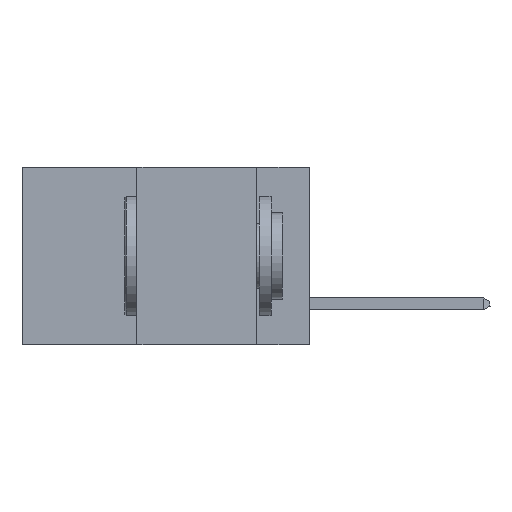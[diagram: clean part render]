
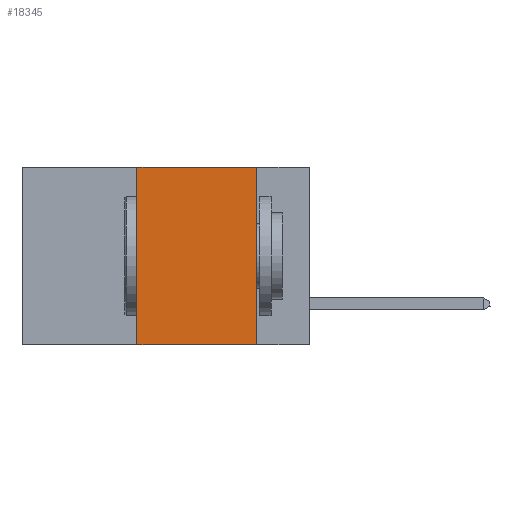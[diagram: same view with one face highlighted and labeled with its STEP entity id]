
A CAD part, left-side view. The second image highlights one B-rep face of the part: STEP entity #18345.
In plain terms, the highlighted planar face has unit normal (-1, 0, 0).
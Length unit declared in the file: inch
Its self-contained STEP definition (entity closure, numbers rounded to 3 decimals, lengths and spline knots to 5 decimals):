
#171 = VERTEX_POINT ( 'NONE', #15645 ) ;
#567 = CARTESIAN_POINT ( 'NONE',  ( 0., 0.36, 0. ) ) ;
#856 = CARTESIAN_POINT ( 'NONE',  ( 0., 0.6, 0. ) ) ;
#2306 = ORIENTED_EDGE ( 'NONE', *, *, #4148, .F. ) ;
#2376 = EDGE_LOOP ( 'NONE', ( #21648, #2306, #12618, #24026 ) ) ;
#2383 = LINE ( 'NONE', #19832, #6297 ) ;
#2520 = DIRECTION ( 'NONE',  ( 0., 0., 1. ) ) ;
#2818 = DIRECTION ( 'NONE',  ( 0., 0., -1. ) ) ;
#4148 = EDGE_CURVE ( 'NONE', #15602, #171, #2383, .T. ) ;
#4339 = CARTESIAN_POINT ( 'NONE',  ( 0., 0.11, 0. ) ) ;
#4384 = VERTEX_POINT ( 'NONE', #9303 ) ;
#5113 = CARTESIAN_POINT ( 'NONE',  ( 0., 0.6, -0.37 ) ) ;
#6297 = VECTOR ( 'NONE', #19319, 39.37008 ) ;
#7055 = DIRECTION ( 'NONE',  ( 0., -1., 0. ) ) ;
#9303 = CARTESIAN_POINT ( 'NONE',  ( 0., 0.11, -0.37 ) ) ;
#9849 = EDGE_CURVE ( 'NONE', #18872, #4384, #13884, .T. ) ;
#10145 = AXIS2_PLACEMENT_3D ( 'NONE', #856, #14444, #2818 ) ;
#11339 = EDGE_CURVE ( 'NONE', #18872, #15602, #24880, .T. ) ;
#12463 = CARTESIAN_POINT ( 'NONE',  ( 0., 0.36, -0.37 ) ) ;
#12618 = ORIENTED_EDGE ( 'NONE', *, *, #11339, .F. ) ;
#13273 = VECTOR ( 'NONE', #7055, 39.37008 ) ;
#13844 = VECTOR ( 'NONE', #2520, 39.37008 ) ;
#13884 = LINE ( 'NONE', #5113, #13273 ) ;
#14359 = FACE_OUTER_BOUND ( 'NONE', #2376, .T. ) ;
#14444 = DIRECTION ( 'NONE',  ( 1., 0., 0. ) ) ;
#15079 = EDGE_CURVE ( 'NONE', #171, #4384, #20224, .T. ) ;
#15127 = VECTOR ( 'NONE', #21736, 39.37008 ) ;
#15602 = VERTEX_POINT ( 'NONE', #24952 ) ;
#15645 = CARTESIAN_POINT ( 'NONE',  ( 0., 0.11, 0. ) ) ;
#18345 = ADVANCED_FACE ( 'NONE', ( #14359 ), #22078, .F. ) ;
#18872 = VERTEX_POINT ( 'NONE', #12463 ) ;
#19319 = DIRECTION ( 'NONE',  ( 0., -1., 0. ) ) ;
#19832 = CARTESIAN_POINT ( 'NONE',  ( 0., 0.6, 0. ) ) ;
#20224 = LINE ( 'NONE', #4339, #15127 ) ;
#21648 = ORIENTED_EDGE ( 'NONE', *, *, #15079, .F. ) ;
#21736 = DIRECTION ( 'NONE',  ( 0., 0., -1. ) ) ;
#22078 = PLANE ( 'NONE',  #10145 ) ;
#24026 = ORIENTED_EDGE ( 'NONE', *, *, #9849, .T. ) ;
#24880 = LINE ( 'NONE', #567, #13844 ) ;
#24952 = CARTESIAN_POINT ( 'NONE',  ( 0., 0.36, 0. ) ) ;
